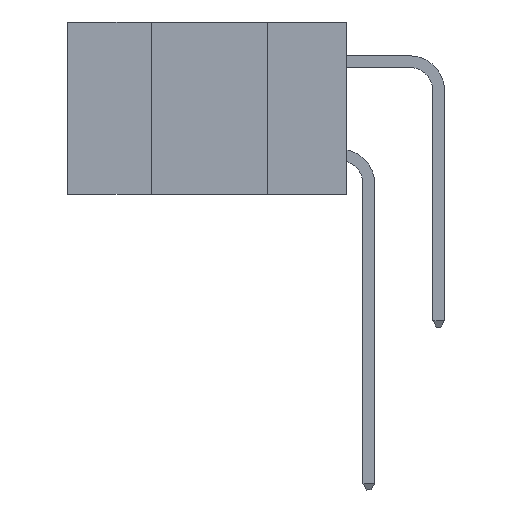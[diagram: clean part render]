
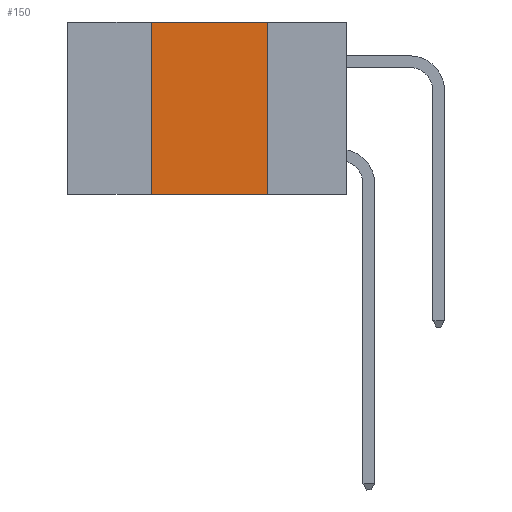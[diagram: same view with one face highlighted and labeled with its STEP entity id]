
A CAD part, left-side view. The second image highlights one B-rep face of the part: STEP entity #150.
In plain terms, the highlighted planar face has unit normal (-1, 0, 0).
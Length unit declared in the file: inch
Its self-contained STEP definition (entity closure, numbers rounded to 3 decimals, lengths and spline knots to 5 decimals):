
#40 = VECTOR ( 'NONE', #1969, 39.37008 ) ;
#150 = ADVANCED_FACE ( 'NONE', ( #10470 ), #1569, .F. ) ;
#488 = CARTESIAN_POINT ( 'NONE',  ( 0., 0.42, 0. ) ) ;
#622 = VERTEX_POINT ( 'NONE', #12024 ) ;
#1569 = PLANE ( 'NONE',  #3467 ) ;
#1969 = DIRECTION ( 'NONE',  ( 0., 0., -1. ) ) ;
#2184 = VERTEX_POINT ( 'NONE', #488 ) ;
#2528 = LINE ( 'NONE', #4967, #9829 ) ;
#3467 = AXIS2_PLACEMENT_3D ( 'NONE', #5804, #5457, #4381 ) ;
#3914 = CARTESIAN_POINT ( 'NONE',  ( 0., 0.17, 0. ) ) ;
#4179 = ORIENTED_EDGE ( 'NONE', *, *, #8034, .T. ) ;
#4284 = DIRECTION ( 'NONE',  ( 0., -1., 0. ) ) ;
#4311 = CARTESIAN_POINT ( 'NONE',  ( 0., 0.17, 0. ) ) ;
#4381 = DIRECTION ( 'NONE',  ( 0., 0., -1. ) ) ;
#4967 = CARTESIAN_POINT ( 'NONE',  ( 0., 0.42, 0. ) ) ;
#5216 = CARTESIAN_POINT ( 'NONE',  ( 0., 0.6, -0.37 ) ) ;
#5457 = DIRECTION ( 'NONE',  ( 1., 0., 0. ) ) ;
#5630 = LINE ( 'NONE', #3914, #40 ) ;
#5804 = CARTESIAN_POINT ( 'NONE',  ( 0., 0.6, 0. ) ) ;
#6157 = EDGE_LOOP ( 'NONE', ( #11929, #6697, #12229, #4179 ) ) ;
#6224 = DIRECTION ( 'NONE',  ( 0., -1., 0. ) ) ;
#6658 = CARTESIAN_POINT ( 'NONE',  ( 0., 0.17, -0.37 ) ) ;
#6697 = ORIENTED_EDGE ( 'NONE', *, *, #9576, .F. ) ;
#6800 = VERTEX_POINT ( 'NONE', #4311 ) ;
#7174 = EDGE_CURVE ( 'NONE', #622, #2184, #2528, .T. ) ;
#7872 = VECTOR ( 'NONE', #6224, 39.37008 ) ;
#8034 = EDGE_CURVE ( 'NONE', #622, #10649, #8791, .T. ) ;
#8121 = CARTESIAN_POINT ( 'NONE',  ( 0., 0.6, 0. ) ) ;
#8190 = VECTOR ( 'NONE', #4284, 39.37008 ) ;
#8791 = LINE ( 'NONE', #5216, #8190 ) ;
#9576 = EDGE_CURVE ( 'NONE', #2184, #6800, #10315, .T. ) ;
#9687 = DIRECTION ( 'NONE',  ( 0., 0., 1. ) ) ;
#9829 = VECTOR ( 'NONE', #9687, 39.37008 ) ;
#9987 = EDGE_CURVE ( 'NONE', #6800, #10649, #5630, .T. ) ;
#10315 = LINE ( 'NONE', #8121, #7872 ) ;
#10470 = FACE_OUTER_BOUND ( 'NONE', #6157, .T. ) ;
#10649 = VERTEX_POINT ( 'NONE', #6658 ) ;
#11929 = ORIENTED_EDGE ( 'NONE', *, *, #9987, .F. ) ;
#12024 = CARTESIAN_POINT ( 'NONE',  ( 0., 0.42, -0.37 ) ) ;
#12229 = ORIENTED_EDGE ( 'NONE', *, *, #7174, .F. ) ;
